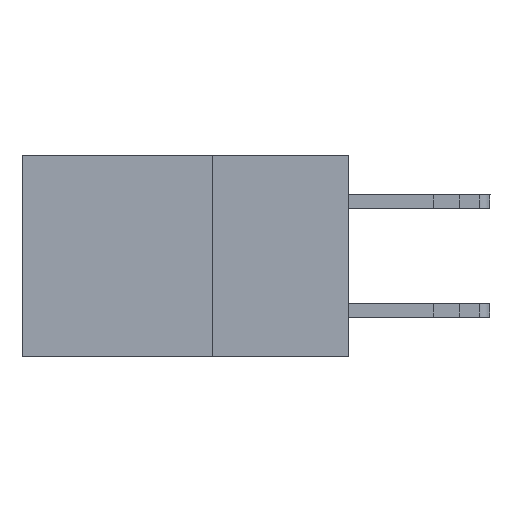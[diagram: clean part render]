
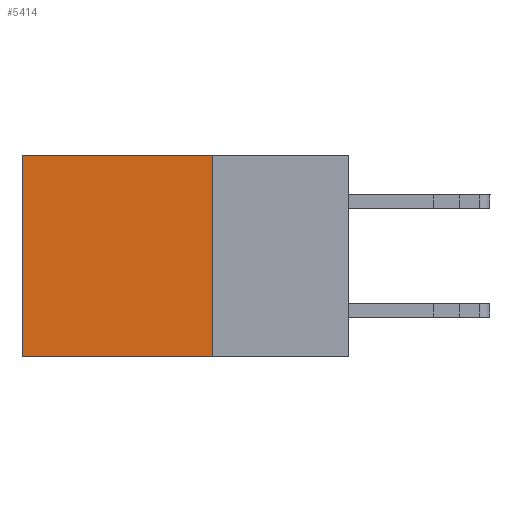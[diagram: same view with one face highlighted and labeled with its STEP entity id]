
A CAD part, left-side view. The second image highlights one B-rep face of the part: STEP entity #5414.
In plain terms, the highlighted planar face has unit normal (-1, 0, 0).
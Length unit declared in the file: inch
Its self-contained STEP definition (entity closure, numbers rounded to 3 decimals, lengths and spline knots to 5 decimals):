
#461 = DIRECTION ( 'NONE',  ( 0., 0., -1. ) ) ;
#527 = DIRECTION ( 'NONE',  ( 1., 0., 0. ) ) ;
#1432 = CARTESIAN_POINT ( 'NONE',  ( 0.298, 0.25, 0. ) ) ;
#2062 = AXIS2_PLACEMENT_3D ( 'NONE', #18774, #527, #461 ) ;
#2447 = DIRECTION ( 'NONE',  ( 0., 0., -1. ) ) ;
#3484 = FACE_OUTER_BOUND ( 'NONE', #16650, .T. ) ;
#3614 = CARTESIAN_POINT ( 'NONE',  ( 0.298, 0.6, 0. ) ) ;
#3835 = CARTESIAN_POINT ( 'NONE',  ( 0.298, 0.6, -0.37 ) ) ;
#5151 = CARTESIAN_POINT ( 'NONE',  ( 0.298, 0.25, 0. ) ) ;
#5414 = ADVANCED_FACE ( 'NONE', ( #3484 ), #17749, .F. ) ;
#5798 = ORIENTED_EDGE ( 'NONE', *, *, #14472, .F. ) ;
#6753 = DIRECTION ( 'NONE',  ( 0., 1., 0. ) ) ;
#7044 = VECTOR ( 'NONE', #9508, 39.37008 ) ;
#8646 = EDGE_CURVE ( 'NONE', #13742, #15544, #16441, .T. ) ;
#8771 = CARTESIAN_POINT ( 'NONE',  ( 0.298, 0.25, 0. ) ) ;
#9169 = DIRECTION ( 'NONE',  ( 0., 0., -1. ) ) ;
#9339 = VERTEX_POINT ( 'NONE', #11091 ) ;
#9442 = CARTESIAN_POINT ( 'NONE',  ( 0.298, 0.25, -0.37 ) ) ;
#9508 = DIRECTION ( 'NONE',  ( 0., 1., 0. ) ) ;
#9515 = LINE ( 'NONE', #8771, #17272 ) ;
#9531 = VECTOR ( 'NONE', #6753, 39.37008 ) ;
#10604 = LINE ( 'NONE', #17857, #14517 ) ;
#11091 = CARTESIAN_POINT ( 'NONE',  ( 0.298, 0.25, -0.37 ) ) ;
#11634 = EDGE_CURVE ( 'NONE', #13742, #9339, #9515, .T. ) ;
#13657 = EDGE_CURVE ( 'NONE', #15544, #19285, #10604, .T. ) ;
#13742 = VERTEX_POINT ( 'NONE', #1432 ) ;
#14472 = EDGE_CURVE ( 'NONE', #9339, #19285, #18725, .T. ) ;
#14517 = VECTOR ( 'NONE', #9169, 39.37008 ) ;
#15544 = VERTEX_POINT ( 'NONE', #3614 ) ;
#15872 = ORIENTED_EDGE ( 'NONE', *, *, #11634, .F. ) ;
#16441 = LINE ( 'NONE', #5151, #9531 ) ;
#16650 = EDGE_LOOP ( 'NONE', ( #19419, #5798, #15872, #18622 ) ) ;
#17272 = VECTOR ( 'NONE', #2447, 39.37008 ) ;
#17749 = PLANE ( 'NONE',  #2062 ) ;
#17857 = CARTESIAN_POINT ( 'NONE',  ( 0.298, 0.6, 0. ) ) ;
#18622 = ORIENTED_EDGE ( 'NONE', *, *, #8646, .T. ) ;
#18725 = LINE ( 'NONE', #9442, #7044 ) ;
#18774 = CARTESIAN_POINT ( 'NONE',  ( 0.298, 0.25, 0. ) ) ;
#19285 = VERTEX_POINT ( 'NONE', #3835 ) ;
#19419 = ORIENTED_EDGE ( 'NONE', *, *, #13657, .T. ) ;
